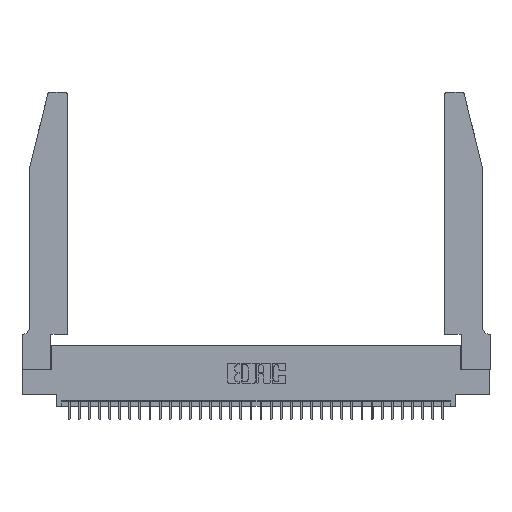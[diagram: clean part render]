
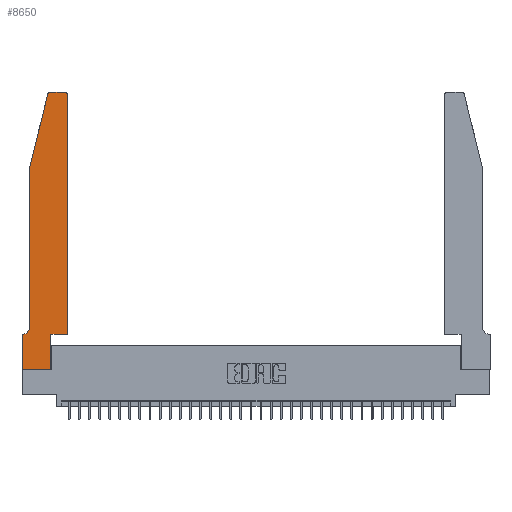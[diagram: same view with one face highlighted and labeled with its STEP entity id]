
A CAD part, top view. The second image highlights one B-rep face of the part: STEP entity #8650.
In plain terms, the highlighted planar face has unit normal (0, 0, 1).
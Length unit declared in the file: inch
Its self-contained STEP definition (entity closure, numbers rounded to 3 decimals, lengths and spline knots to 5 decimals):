
#223 = EDGE_CURVE ( 'NONE', #19917, #4270, #12387, .T. ) ;
#232 = CARTESIAN_POINT ( 'NONE',  ( 0.4505, 0.35, 0.37 ) ) ;
#394 = CARTESIAN_POINT ( 'NONE',  ( 0.0755, 2., 0.37 ) ) ;
#397 = DIRECTION ( 'NONE',  ( 0., 0., 1. ) ) ;
#617 = VECTOR ( 'NONE', #12709, 39.37008 ) ;
#922 = CARTESIAN_POINT ( 'NONE',  ( 0., 0.35, 0.37 ) ) ;
#1366 = ORIENTED_EDGE ( 'NONE', *, *, #14587, .T. ) ;
#1818 = CARTESIAN_POINT ( 'NONE',  ( 0.0055, 0.42, 0.37 ) ) ;
#1842 = LINE ( 'NONE', #23848, #617 ) ;
#2080 = VERTEX_POINT ( 'NONE', #8940 ) ;
#2163 = CARTESIAN_POINT ( 'NONE',  ( 0.4505, 0.35, 0.37 ) ) ;
#2168 = VECTOR ( 'NONE', #34225, 39.37008 ) ;
#2216 = VECTOR ( 'NONE', #9899, 39.37008 ) ;
#2373 = CARTESIAN_POINT ( 'NONE',  ( 0., 0.35, 0.37 ) ) ;
#2562 = CARTESIAN_POINT ( 'NONE',  ( 0.0055, 0.35, 0.37 ) ) ;
#3364 = ORIENTED_EDGE ( 'NONE', *, *, #31498, .T. ) ;
#3634 = VECTOR ( 'NONE', #33404, 39.37008 ) ;
#3742 = CARTESIAN_POINT ( 'NONE',  ( 0.284, 2.72, 0.37 ) ) ;
#4161 = DIRECTION ( 'NONE',  ( 1., 0., 0. ) ) ;
#4270 = VERTEX_POINT ( 'NONE', #6175 ) ;
#5779 = LINE ( 'NONE', #232, #25141 ) ;
#6116 = PLANE ( 'NONE',  #25494 ) ;
#6175 = CARTESIAN_POINT ( 'NONE',  ( 0., 0., 0.37 ) ) ;
#6653 = CARTESIAN_POINT ( 'NONE',  ( 0.0755, 2., 0.37 ) ) ;
#7512 = LINE ( 'NONE', #25938, #16627 ) ;
#7930 = VECTOR ( 'NONE', #23112, 39.37008 ) ;
#8650 = ADVANCED_FACE ( 'NONE', ( #33149 ), #6116, .T. ) ;
#8775 = DIRECTION ( 'NONE',  ( 0., 1., 0. ) ) ;
#8877 = ORIENTED_EDGE ( 'NONE', *, *, #13470, .T. ) ;
#8940 = CARTESIAN_POINT ( 'NONE',  ( 0.2865, 0., 0.37 ) ) ;
#9259 = CARTESIAN_POINT ( 'NONE',  ( 0.284, 2.75, 0.37 ) ) ;
#9730 = CIRCLE ( 'NONE', #18876, 0.03 ) ;
#9899 = DIRECTION ( 'NONE',  ( 0., -1., 0. ) ) ;
#10184 = AXIS2_PLACEMENT_3D ( 'NONE', #1818, #26837, #13041 ) ;
#10729 = VECTOR ( 'NONE', #22222, 39.37008 ) ;
#11399 = LINE ( 'NONE', #30545, #3634 ) ;
#11663 = CARTESIAN_POINT ( 'NONE',  ( 0.4205, 2.72, 0.37 ) ) ;
#12260 = ORIENTED_EDGE ( 'NONE', *, *, #223, .T. ) ;
#12387 = LINE ( 'NONE', #18325, #2216 ) ;
#12668 = CARTESIAN_POINT ( 'NONE',  ( 0.0755, 0.42, 0.37 ) ) ;
#12709 = DIRECTION ( 'NONE',  ( -1., 0., 0. ) ) ;
#13041 = DIRECTION ( 'NONE',  ( -1., 0., 0. ) ) ;
#13100 = DIRECTION ( 'NONE',  ( 0., 1., 0. ) ) ;
#13470 = EDGE_CURVE ( 'NONE', #20817, #13890, #21586, .T. ) ;
#13496 = VERTEX_POINT ( 'NONE', #23956 ) ;
#13582 = CIRCLE ( 'NONE', #10184, 0.07 ) ;
#13890 = VERTEX_POINT ( 'NONE', #17818 ) ;
#13962 = LINE ( 'NONE', #394, #10729 ) ;
#13968 = ORIENTED_EDGE ( 'NONE', *, *, #28758, .T. ) ;
#14587 = EDGE_CURVE ( 'NONE', #13890, #27814, #33653, .T. ) ;
#14701 = ORIENTED_EDGE ( 'NONE', *, *, #15869, .T. ) ;
#14839 = CARTESIAN_POINT ( 'NONE',  ( 0.2865, 0.35, 0.37 ) ) ;
#15417 = CARTESIAN_POINT ( 'NONE',  ( 0.4505, 0.35, 0.37 ) ) ;
#15869 = EDGE_CURVE ( 'NONE', #27814, #19159, #13962, .T. ) ;
#16070 = DIRECTION ( 'NONE',  ( -1., 0., 0. ) ) ;
#16076 = VERTEX_POINT ( 'NONE', #2163 ) ;
#16136 = EDGE_CURVE ( 'NONE', #19159, #17596, #13582, .T. ) ;
#16627 = VECTOR ( 'NONE', #16070, 39.37008 ) ;
#16996 = LINE ( 'NONE', #14839, #29815 ) ;
#17133 = ORIENTED_EDGE ( 'NONE', *, *, #20265, .T. ) ;
#17596 = VERTEX_POINT ( 'NONE', #2562 ) ;
#17818 = CARTESIAN_POINT ( 'NONE',  ( 0.25487, 2.72718, 0.37 ) ) ;
#17884 = CARTESIAN_POINT ( 'NONE',  ( 0.4205, 2.75, 0.37 ) ) ;
#18320 = ORIENTED_EDGE ( 'NONE', *, *, #32006, .T. ) ;
#18325 = CARTESIAN_POINT ( 'NONE',  ( 0., 0., 0.37 ) ) ;
#18584 = EDGE_CURVE ( 'NONE', #13496, #28161, #9730, .T. ) ;
#18876 = AXIS2_PLACEMENT_3D ( 'NONE', #11663, #25810, #4161 ) ;
#19159 = VERTEX_POINT ( 'NONE', #12668 ) ;
#19866 = EDGE_LOOP ( 'NONE', ( #18320, #8877, #1366, #14701, #20926, #3364, #12260, #30015, #17133, #33077, #13968, #23904 ) ) ;
#19917 = VERTEX_POINT ( 'NONE', #2373 ) ;
#20265 = EDGE_CURVE ( 'NONE', #2080, #30401, #16996, .T. ) ;
#20817 = VERTEX_POINT ( 'NONE', #9259 ) ;
#20926 = ORIENTED_EDGE ( 'NONE', *, *, #16136, .T. ) ;
#21586 = CIRCLE ( 'NONE', #27875, 0.03 ) ;
#22222 = DIRECTION ( 'NONE',  ( 0., -1., 0. ) ) ;
#22480 = EDGE_CURVE ( 'NONE', #4270, #2080, #11399, .T. ) ;
#23112 = DIRECTION ( 'NONE',  ( -0.239, -0.971, 0. ) ) ;
#23331 = LINE ( 'NONE', #15417, #2168 ) ;
#23848 = CARTESIAN_POINT ( 'NONE',  ( 0.0755, 0.35, 0.37 ) ) ;
#23904 = ORIENTED_EDGE ( 'NONE', *, *, #18584, .T. ) ;
#23956 = CARTESIAN_POINT ( 'NONE',  ( 0.4505, 2.72, 0.37 ) ) ;
#25141 = VECTOR ( 'NONE', #13100, 39.37008 ) ;
#25494 = AXIS2_PLACEMENT_3D ( 'NONE', #922, #397, #27947 ) ;
#25810 = DIRECTION ( 'NONE',  ( 0., 0., 1. ) ) ;
#25938 = CARTESIAN_POINT ( 'NONE',  ( 0.2605, 2.75, 0.37 ) ) ;
#25993 = EDGE_CURVE ( 'NONE', #30401, #16076, #23331, .T. ) ;
#26837 = DIRECTION ( 'NONE',  ( 0., 0., -1. ) ) ;
#27814 = VERTEX_POINT ( 'NONE', #6653 ) ;
#27875 = AXIS2_PLACEMENT_3D ( 'NONE', #3742, #31474, #30743 ) ;
#27947 = DIRECTION ( 'NONE',  ( 1., 0., 0. ) ) ;
#28161 = VERTEX_POINT ( 'NONE', #17884 ) ;
#28407 = CARTESIAN_POINT ( 'NONE',  ( 0.2865, 0.35, 0.37 ) ) ;
#28758 = EDGE_CURVE ( 'NONE', #16076, #13496, #5779, .T. ) ;
#29815 = VECTOR ( 'NONE', #8775, 39.37008 ) ;
#30015 = ORIENTED_EDGE ( 'NONE', *, *, #22480, .T. ) ;
#30401 = VERTEX_POINT ( 'NONE', #28407 ) ;
#30545 = CARTESIAN_POINT ( 'NONE',  ( 0., 0., 0.37 ) ) ;
#30743 = DIRECTION ( 'NONE',  ( 1., 0., 0. ) ) ;
#31135 = CARTESIAN_POINT ( 'NONE',  ( 0.0755, 2., 0.37 ) ) ;
#31474 = DIRECTION ( 'NONE',  ( 0., 0., 1. ) ) ;
#31498 = EDGE_CURVE ( 'NONE', #17596, #19917, #1842, .T. ) ;
#32006 = EDGE_CURVE ( 'NONE', #28161, #20817, #7512, .T. ) ;
#33077 = ORIENTED_EDGE ( 'NONE', *, *, #25993, .T. ) ;
#33149 = FACE_OUTER_BOUND ( 'NONE', #19866, .T. ) ;
#33404 = DIRECTION ( 'NONE',  ( 1., 0., 0. ) ) ;
#33653 = LINE ( 'NONE', #31135, #7930 ) ;
#34225 = DIRECTION ( 'NONE',  ( 1., 0., 0. ) ) ;
